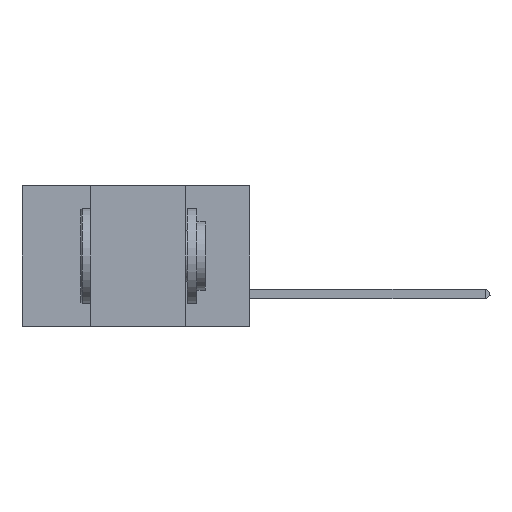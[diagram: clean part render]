
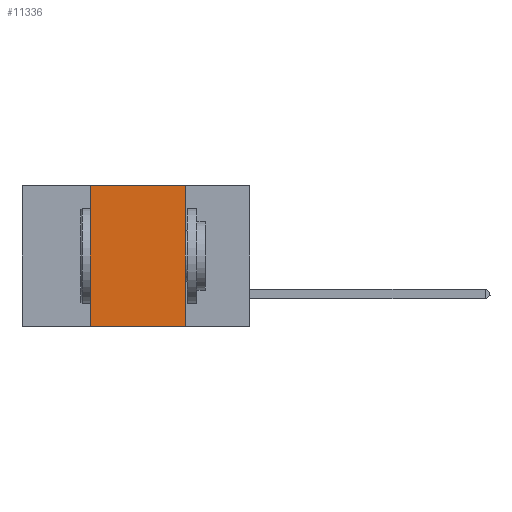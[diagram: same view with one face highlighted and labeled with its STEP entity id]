
A CAD part, left-side view. The second image highlights one B-rep face of the part: STEP entity #11336.
In plain terms, the highlighted planar face has unit normal (-1, 0, 0).
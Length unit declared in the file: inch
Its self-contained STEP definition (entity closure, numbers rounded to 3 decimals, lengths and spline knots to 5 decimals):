
#763 = PLANE ( 'NONE',  #25199 ) ;
#964 = DIRECTION ( 'NONE',  ( 0., -1., 0. ) ) ;
#2354 = EDGE_CURVE ( 'NONE', #9573, #4582, #15036, .T. ) ;
#3081 = DIRECTION ( 'NONE',  ( 0., -1., 0. ) ) ;
#3591 = LINE ( 'NONE', #8859, #23787 ) ;
#3596 = VECTOR ( 'NONE', #964, 39.37008 ) ;
#4436 = VERTEX_POINT ( 'NONE', #4624 ) ;
#4438 = VECTOR ( 'NONE', #14504, 39.37008 ) ;
#4582 = VERTEX_POINT ( 'NONE', #11109 ) ;
#4624 = CARTESIAN_POINT ( 'NONE',  ( 0., 0.17, -0.37 ) ) ;
#7577 = CARTESIAN_POINT ( 'NONE',  ( 0., 0.42, 0. ) ) ;
#8799 = CARTESIAN_POINT ( 'NONE',  ( 0., 0.42, -0.37 ) ) ;
#8859 = CARTESIAN_POINT ( 'NONE',  ( 0., 0.6, -0.37 ) ) ;
#9573 = VERTEX_POINT ( 'NONE', #7577 ) ;
#10646 = ORIENTED_EDGE ( 'NONE', *, *, #2354, .F. ) ;
#11007 = CARTESIAN_POINT ( 'NONE',  ( 0., 0.6, 0. ) ) ;
#11109 = CARTESIAN_POINT ( 'NONE',  ( 0., 0.17, 0. ) ) ;
#11336 = ADVANCED_FACE ( 'NONE', ( #14353 ), #763, .F. ) ;
#14353 = FACE_OUTER_BOUND ( 'NONE', #14591, .T. ) ;
#14504 = DIRECTION ( 'NONE',  ( 0., 0., -1. ) ) ;
#14591 = EDGE_LOOP ( 'NONE', ( #20448, #10646, #15934, #18798 ) ) ;
#14777 = CARTESIAN_POINT ( 'NONE',  ( 0., 0.17, 0. ) ) ;
#15036 = LINE ( 'NONE', #11007, #3596 ) ;
#15934 = ORIENTED_EDGE ( 'NONE', *, *, #19697, .F. ) ;
#16035 = EDGE_CURVE ( 'NONE', #23451, #4436, #3591, .T. ) ;
#18268 = VECTOR ( 'NONE', #26213, 39.37008 ) ;
#18798 = ORIENTED_EDGE ( 'NONE', *, *, #16035, .T. ) ;
#19010 = CARTESIAN_POINT ( 'NONE',  ( 0., 0.6, 0. ) ) ;
#19697 = EDGE_CURVE ( 'NONE', #23451, #9573, #23613, .T. ) ;
#20214 = CARTESIAN_POINT ( 'NONE',  ( 0., 0.42, 0. ) ) ;
#20448 = ORIENTED_EDGE ( 'NONE', *, *, #24031, .F. ) ;
#21030 = DIRECTION ( 'NONE',  ( 0., 0., -1. ) ) ;
#21111 = DIRECTION ( 'NONE',  ( 1., 0., 0. ) ) ;
#21486 = LINE ( 'NONE', #14777, #4438 ) ;
#23451 = VERTEX_POINT ( 'NONE', #8799 ) ;
#23613 = LINE ( 'NONE', #20214, #18268 ) ;
#23787 = VECTOR ( 'NONE', #3081, 39.37008 ) ;
#24031 = EDGE_CURVE ( 'NONE', #4582, #4436, #21486, .T. ) ;
#25199 = AXIS2_PLACEMENT_3D ( 'NONE', #19010, #21111, #21030 ) ;
#26213 = DIRECTION ( 'NONE',  ( 0., 0., 1. ) ) ;
